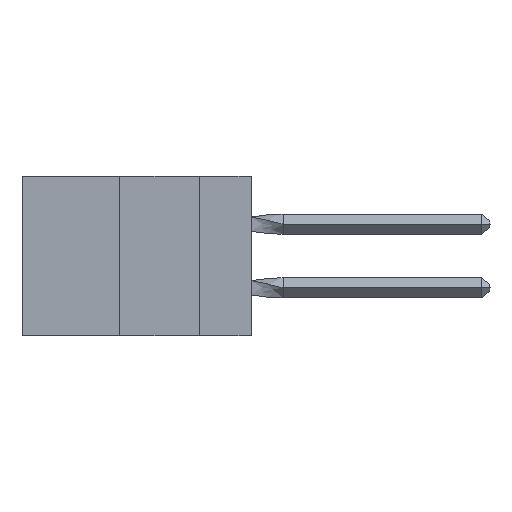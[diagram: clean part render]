
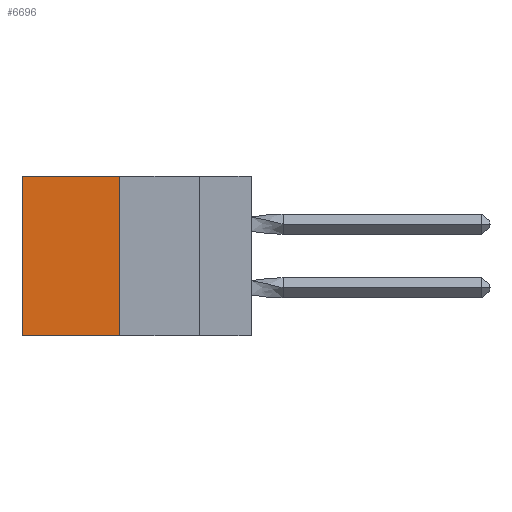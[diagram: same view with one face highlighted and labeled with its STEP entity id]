
A CAD part, left-side view. The second image highlights one B-rep face of the part: STEP entity #6696.
In plain terms, the highlighted planar face has unit normal (-1, 0, 0).
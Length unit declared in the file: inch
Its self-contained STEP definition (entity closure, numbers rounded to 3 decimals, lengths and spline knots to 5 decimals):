
#1333 = CARTESIAN_POINT ( 'NONE',  ( 0.305, 0.413, -0.5 ) ) ;
#1419 = DIRECTION ( 'NONE',  ( 0., 1., 0. ) ) ;
#2464 = VERTEX_POINT ( 'NONE', #18051 ) ;
#3011 = LINE ( 'NONE', #25153, #3312 ) ;
#3208 = PLANE ( 'NONE',  #22388 ) ;
#3312 = VECTOR ( 'NONE', #25327, 39.37008 ) ;
#3386 = EDGE_LOOP ( 'NONE', ( #5726, #8414, #19136, #11702 ) ) ;
#3723 = CARTESIAN_POINT ( 'NONE',  ( 0.305, 0.72, -0.5 ) ) ;
#3810 = DIRECTION ( 'NONE',  ( 0., 0., -1. ) ) ;
#5225 = CARTESIAN_POINT ( 'NONE',  ( 0.305, 0.413, 0. ) ) ;
#5442 = CARTESIAN_POINT ( 'NONE',  ( 0.305, 0.413, 0. ) ) ;
#5726 = ORIENTED_EDGE ( 'NONE', *, *, #17134, .T. ) ;
#6696 = ADVANCED_FACE ( 'NONE', ( #24265 ), #3208, .F. ) ;
#8414 = ORIENTED_EDGE ( 'NONE', *, *, #24936, .F. ) ;
#8998 = EDGE_CURVE ( 'NONE', #23789, #2464, #24175, .T. ) ;
#10939 = DIRECTION ( 'NONE',  ( 0., 0., -1. ) ) ;
#11207 = VECTOR ( 'NONE', #22424, 39.37008 ) ;
#11702 = ORIENTED_EDGE ( 'NONE', *, *, #8998, .T. ) ;
#13014 = CARTESIAN_POINT ( 'NONE',  ( 0.305, 0.413, -0.5 ) ) ;
#17134 = EDGE_CURVE ( 'NONE', #2464, #23928, #21774, .T. ) ;
#18051 = CARTESIAN_POINT ( 'NONE',  ( 0.305, 0.72, 0. ) ) ;
#18528 = LINE ( 'NONE', #24478, #11207 ) ;
#19136 = ORIENTED_EDGE ( 'NONE', *, *, #20020, .F. ) ;
#19769 = VERTEX_POINT ( 'NONE', #13014 ) ;
#20020 = EDGE_CURVE ( 'NONE', #23789, #19769, #3011, .T. ) ;
#20658 = DIRECTION ( 'NONE',  ( 1., 0., 0. ) ) ;
#20817 = VECTOR ( 'NONE', #1419, 39.37008 ) ;
#21774 = LINE ( 'NONE', #23709, #23288 ) ;
#22388 = AXIS2_PLACEMENT_3D ( 'NONE', #1333, #20658, #10939 ) ;
#22424 = DIRECTION ( 'NONE',  ( 0., 1., 0. ) ) ;
#23288 = VECTOR ( 'NONE', #3810, 39.37008 ) ;
#23709 = CARTESIAN_POINT ( 'NONE',  ( 0.305, 0.72, -0.5 ) ) ;
#23789 = VERTEX_POINT ( 'NONE', #5225 ) ;
#23928 = VERTEX_POINT ( 'NONE', #3723 ) ;
#24175 = LINE ( 'NONE', #5442, #20817 ) ;
#24265 = FACE_OUTER_BOUND ( 'NONE', #3386, .T. ) ;
#24478 = CARTESIAN_POINT ( 'NONE',  ( 0.305, 0.413, -0.5 ) ) ;
#24936 = EDGE_CURVE ( 'NONE', #19769, #23928, #18528, .T. ) ;
#25153 = CARTESIAN_POINT ( 'NONE',  ( 0.305, 0.413, -0.5 ) ) ;
#25327 = DIRECTION ( 'NONE',  ( 0., 0., -1. ) ) ;
